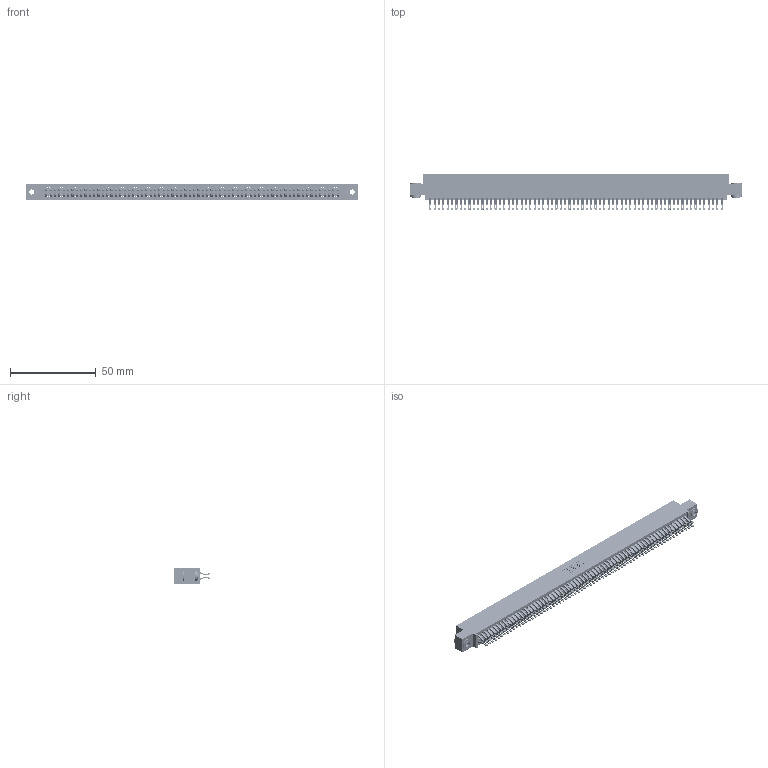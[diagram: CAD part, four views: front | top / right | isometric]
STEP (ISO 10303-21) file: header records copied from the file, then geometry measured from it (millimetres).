
FILE_DESCRIPTION (( 'STEP AP203' ), '1' );
FILE_NAME ('395-136-555-503.STEP', '2018-12-05T10:11:57', ( '' ), ( '' ), 'SwSTEP 2.0', 'SolidWorks 2016', '' );
FILE_SCHEMA (( 'CONFIG_CONTROL_DESIGN' ));
Length unit declared in the file: inch
Products named in the file (4): 395-136-555-503; 345 Part_0.110 Offset - 0.156 Dia-TH; 345-292-001_555 Tail; 345-250-002_345-250-002-102
Assembly tree (139 placements, depth 2):
  395-136-555-503
    345 Part_0.110 Offset - 0.156 Dia-TH
    345-292-001_555 Tail  x136
    345-250-002_345-250-002-102  x2
Bounding box: 193.93 x 21.13 x 9.4 mm (x, y, z)
Volume: 19420.3 mm3; surface area: 30879.8 mm2
Topology: 139 solids, 139 shells, 7784 faces, 24501 edges, 16330 vertices
Faces by surface type: plane 4310, cylinder 3466, cone 8
Entity records: 50962 total; most frequent: CARTESIAN_POINT 8529, ORIENTED_EDGE 8426, DIRECTION 7487, EDGE_CURVE 4213, LINE 3765, VECTOR 3765, VERTEX_POINT 2806, AXIS2_PLACEMENT_3D 1861
